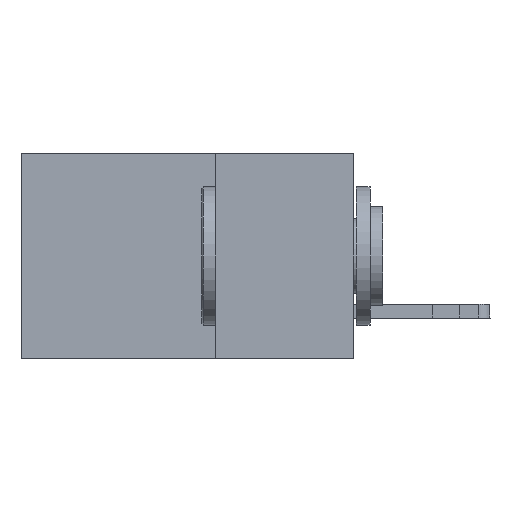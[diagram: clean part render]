
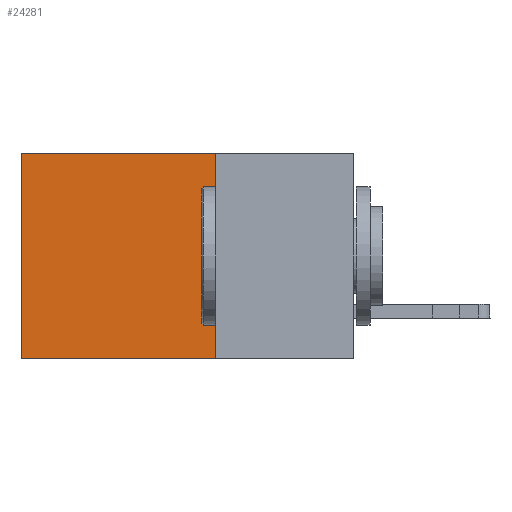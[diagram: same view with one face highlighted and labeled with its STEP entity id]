
A CAD part, left-side view. The second image highlights one B-rep face of the part: STEP entity #24281.
In plain terms, the highlighted planar face has unit normal (-1, 0, 0).
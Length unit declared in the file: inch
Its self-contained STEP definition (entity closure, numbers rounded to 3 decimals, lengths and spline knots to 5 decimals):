
#535 = EDGE_LOOP ( 'NONE', ( #6143, #12234, #27789, #17418 ) ) ;
#1138 = CARTESIAN_POINT ( 'NONE',  ( 0.2875, 0.25, -0.37 ) ) ;
#1973 = CARTESIAN_POINT ( 'NONE',  ( 0.2875, 0.6, 0. ) ) ;
#2447 = DIRECTION ( 'NONE',  ( 0., 0., -1. ) ) ;
#4817 = CARTESIAN_POINT ( 'NONE',  ( 0.2875, 0.6, 0. ) ) ;
#5219 = VECTOR ( 'NONE', #8851, 39.37008 ) ;
#5510 = AXIS2_PLACEMENT_3D ( 'NONE', #6293, #28307, #2447 ) ;
#5962 = FACE_OUTER_BOUND ( 'NONE', #535, .T. ) ;
#6143 = ORIENTED_EDGE ( 'NONE', *, *, #25527, .T. ) ;
#6293 = CARTESIAN_POINT ( 'NONE',  ( 0.2875, 0.25, 0. ) ) ;
#6308 = VERTEX_POINT ( 'NONE', #4817 ) ;
#6373 = DIRECTION ( 'NONE',  ( 0., 0., -1. ) ) ;
#6877 = DIRECTION ( 'NONE',  ( 0., 0., -1. ) ) ;
#8639 = LINE ( 'NONE', #1973, #23404 ) ;
#8851 = DIRECTION ( 'NONE',  ( 0., 1., 0. ) ) ;
#10671 = LINE ( 'NONE', #25744, #27180 ) ;
#12177 = EDGE_CURVE ( 'NONE', #14756, #14173, #12298, .T. ) ;
#12234 = ORIENTED_EDGE ( 'NONE', *, *, #15937, .F. ) ;
#12298 = LINE ( 'NONE', #13431, #28139 ) ;
#12786 = DIRECTION ( 'NONE',  ( 0., 1., 0. ) ) ;
#13431 = CARTESIAN_POINT ( 'NONE',  ( 0.2875, 0.25, 0. ) ) ;
#14173 = VERTEX_POINT ( 'NONE', #1138 ) ;
#14756 = VERTEX_POINT ( 'NONE', #17983 ) ;
#15937 = EDGE_CURVE ( 'NONE', #14173, #16572, #22073, .T. ) ;
#16572 = VERTEX_POINT ( 'NONE', #21332 ) ;
#17418 = ORIENTED_EDGE ( 'NONE', *, *, #26070, .T. ) ;
#17821 = CARTESIAN_POINT ( 'NONE',  ( 0.2875, 0.25, -0.37 ) ) ;
#17983 = CARTESIAN_POINT ( 'NONE',  ( 0.2875, 0.25, 0. ) ) ;
#21332 = CARTESIAN_POINT ( 'NONE',  ( 0.2875, 0.6, -0.37 ) ) ;
#22073 = LINE ( 'NONE', #17821, #5219 ) ;
#22309 = PLANE ( 'NONE',  #5510 ) ;
#23404 = VECTOR ( 'NONE', #6373, 39.37008 ) ;
#24281 = ADVANCED_FACE ( 'NONE', ( #5962 ), #22309, .F. ) ;
#25527 = EDGE_CURVE ( 'NONE', #6308, #16572, #8639, .T. ) ;
#25744 = CARTESIAN_POINT ( 'NONE',  ( 0.2875, 0.25, 0. ) ) ;
#26070 = EDGE_CURVE ( 'NONE', #14756, #6308, #10671, .T. ) ;
#27180 = VECTOR ( 'NONE', #12786, 39.37008 ) ;
#27789 = ORIENTED_EDGE ( 'NONE', *, *, #12177, .F. ) ;
#28139 = VECTOR ( 'NONE', #6877, 39.37008 ) ;
#28307 = DIRECTION ( 'NONE',  ( 1., 0., 0. ) ) ;
